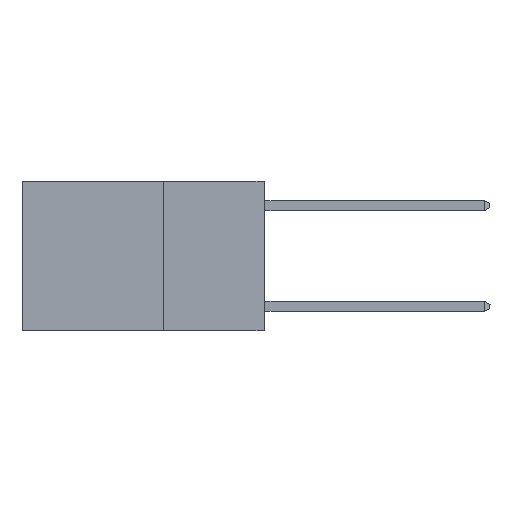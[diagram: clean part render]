
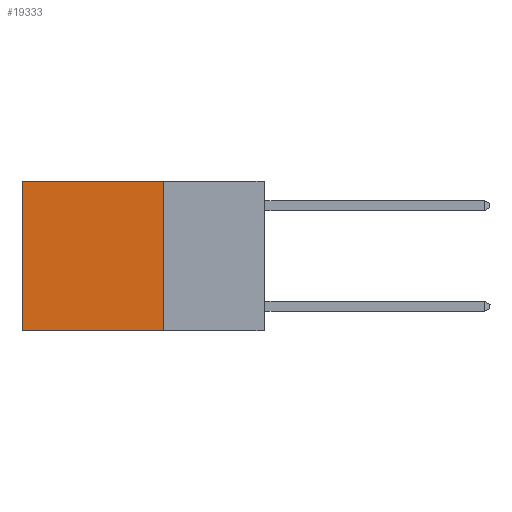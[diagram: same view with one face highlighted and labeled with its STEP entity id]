
A CAD part, left-side view. The second image highlights one B-rep face of the part: STEP entity #19333.
In plain terms, the highlighted planar face has unit normal (-1, 0, 0).
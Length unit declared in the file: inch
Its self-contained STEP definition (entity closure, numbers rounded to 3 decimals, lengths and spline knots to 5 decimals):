
#141 = EDGE_CURVE ( 'NONE', #5340, #5699, #4849, .T. ) ;
#595 = EDGE_CURVE ( 'NONE', #5340, #8661, #20476, .T. ) ;
#1952 = VECTOR ( 'NONE', #14466, 39.37008 ) ;
#2606 = VECTOR ( 'NONE', #13884, 39.37008 ) ;
#2889 = DIRECTION ( 'NONE',  ( 0., 0., -1. ) ) ;
#4054 = CARTESIAN_POINT ( 'NONE',  ( 0.2625, 0.25, 0. ) ) ;
#4849 = LINE ( 'NONE', #8691, #5104 ) ;
#5104 = VECTOR ( 'NONE', #15506, 39.37008 ) ;
#5228 = CARTESIAN_POINT ( 'NONE',  ( 0.2625, 0.25, 0. ) ) ;
#5319 = VERTEX_POINT ( 'NONE', #18696 ) ;
#5321 = ORIENTED_EDGE ( 'NONE', *, *, #17784, .T. ) ;
#5340 = VERTEX_POINT ( 'NONE', #5228 ) ;
#5699 = VERTEX_POINT ( 'NONE', #18575 ) ;
#5949 = DIRECTION ( 'NONE',  ( 1., 0., 0. ) ) ;
#6551 = ORIENTED_EDGE ( 'NONE', *, *, #9988, .F. ) ;
#6915 = LINE ( 'NONE', #21620, #17008 ) ;
#6971 = CARTESIAN_POINT ( 'NONE',  ( 0.2625, 0.25, -0.37 ) ) ;
#8661 = VERTEX_POINT ( 'NONE', #6971 ) ;
#8691 = CARTESIAN_POINT ( 'NONE',  ( 0.2625, 0.25, 0. ) ) ;
#9988 = EDGE_CURVE ( 'NONE', #8661, #5319, #15826, .T. ) ;
#11057 = CARTESIAN_POINT ( 'NONE',  ( 0.2625, 0.25, 0. ) ) ;
#12038 = CARTESIAN_POINT ( 'NONE',  ( 0.2625, 0.25, -0.37 ) ) ;
#12428 = FACE_OUTER_BOUND ( 'NONE', #19169, .T. ) ;
#12869 = DIRECTION ( 'NONE',  ( 0., 0., -1. ) ) ;
#13884 = DIRECTION ( 'NONE',  ( 0., 1., 0. ) ) ;
#14466 = DIRECTION ( 'NONE',  ( 0., 0., -1. ) ) ;
#15506 = DIRECTION ( 'NONE',  ( 0., 1., 0. ) ) ;
#15826 = LINE ( 'NONE', #12038, #2606 ) ;
#15970 = AXIS2_PLACEMENT_3D ( 'NONE', #11057, #5949, #12869 ) ;
#17008 = VECTOR ( 'NONE', #2889, 39.37008 ) ;
#17024 = ORIENTED_EDGE ( 'NONE', *, *, #595, .F. ) ;
#17784 = EDGE_CURVE ( 'NONE', #5699, #5319, #6915, .T. ) ;
#18096 = PLANE ( 'NONE',  #15970 ) ;
#18575 = CARTESIAN_POINT ( 'NONE',  ( 0.2625, 0.6, 0. ) ) ;
#18696 = CARTESIAN_POINT ( 'NONE',  ( 0.2625, 0.6, -0.37 ) ) ;
#19169 = EDGE_LOOP ( 'NONE', ( #5321, #6551, #17024, #21672 ) ) ;
#19333 = ADVANCED_FACE ( 'NONE', ( #12428 ), #18096, .F. ) ;
#20476 = LINE ( 'NONE', #4054, #1952 ) ;
#21620 = CARTESIAN_POINT ( 'NONE',  ( 0.2625, 0.6, 0. ) ) ;
#21672 = ORIENTED_EDGE ( 'NONE', *, *, #141, .T. ) ;
